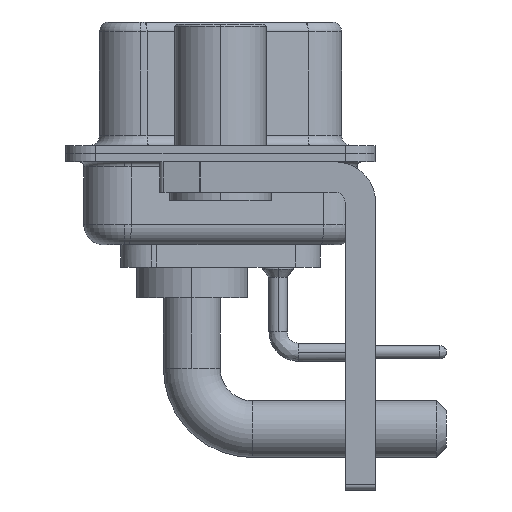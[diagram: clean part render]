
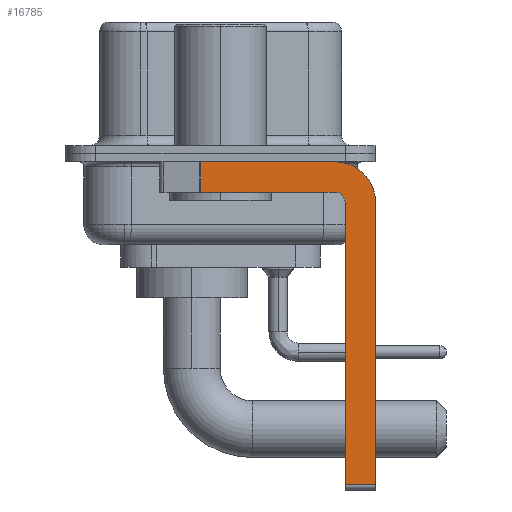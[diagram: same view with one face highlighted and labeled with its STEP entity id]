
A CAD part, left-side view. The second image highlights one B-rep face of the part: STEP entity #16785.
In plain terms, the highlighted planar face has unit normal (-1, 0, 0).
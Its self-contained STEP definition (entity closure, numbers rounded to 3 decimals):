
#169 = CARTESIAN_POINT ( 'NONE',  ( -2.9, -7.65, -16.35 ) ) ;
#586 = DIRECTION ( 'NONE',  ( 0., -1., 0. ) ) ;
#733 = DIRECTION ( 'NONE',  ( 0., 0., -1. ) ) ;
#1070 = VECTOR ( 'NONE', #16345, 1000. ) ;
#1624 = DIRECTION ( 'NONE',  ( 0., 0., -1. ) ) ;
#1710 = LINE ( 'NONE', #3840, #11316 ) ;
#1720 = ORIENTED_EDGE ( 'NONE', *, *, #25575, .F. ) ;
#1809 = VERTEX_POINT ( 'NONE', #169 ) ;
#1882 = LINE ( 'NONE', #2007, #3145 ) ;
#2007 = CARTESIAN_POINT ( 'NONE',  ( -2.9, 0.978, -1.9 ) ) ;
#2187 = LINE ( 'NONE', #10074, #1070 ) ;
#2550 = DIRECTION ( 'NONE',  ( 0., 0., -1. ) ) ;
#2875 = CARTESIAN_POINT ( 'NONE',  ( -2.9, 0.978, -1.9 ) ) ;
#2975 = EDGE_CURVE ( 'NONE', #8226, #8462, #8981, .T. ) ;
#3145 = VECTOR ( 'NONE', #1624, 1000. ) ;
#3410 = EDGE_CURVE ( 'NONE', #8462, #1809, #12719, .T. ) ;
#3652 = ORIENTED_EDGE ( 'NONE', *, *, #23376, .F. ) ;
#3840 = CARTESIAN_POINT ( 'NONE',  ( -2.9, -6.15, -16.6 ) ) ;
#4251 = VERTEX_POINT ( 'NONE', #16491 ) ;
#4537 = CARTESIAN_POINT ( 'NONE',  ( -2.9, -5.65, -1.9 ) ) ;
#4667 = CARTESIAN_POINT ( 'NONE',  ( -2.9, -5.65, -2.4 ) ) ;
#4694 = ORIENTED_EDGE ( 'NONE', *, *, #2975, .F. ) ;
#4807 = PLANE ( 'NONE',  #24754 ) ;
#5439 = VERTEX_POINT ( 'NONE', #19855 ) ;
#5777 = ORIENTED_EDGE ( 'NONE', *, *, #9506, .T. ) ;
#5947 = EDGE_CURVE ( 'NONE', #5439, #8226, #18345, .T. ) ;
#6827 = VERTEX_POINT ( 'NONE', #14478 ) ;
#7837 = DIRECTION ( 'NONE',  ( 0., 0., 1. ) ) ;
#8226 = VERTEX_POINT ( 'NONE', #11596 ) ;
#8462 = VERTEX_POINT ( 'NONE', #9167 ) ;
#8472 = CARTESIAN_POINT ( 'NONE',  ( -2.9, -5.65, -1.9 ) ) ;
#8522 = EDGE_LOOP ( 'NONE', ( #10389, #18802, #3652, #11098, #1720, #5777, #12373, #4694 ) ) ;
#8981 = CIRCLE ( 'NONE', #19205, 2. ) ;
#9109 = VERTEX_POINT ( 'NONE', #2875 ) ;
#9167 = CARTESIAN_POINT ( 'NONE',  ( -2.9, -7.65, -2.4 ) ) ;
#9506 = EDGE_CURVE ( 'NONE', #4251, #1809, #2187, .T. ) ;
#10074 = CARTESIAN_POINT ( 'NONE',  ( -2.9, -5.65, -16.35 ) ) ;
#10216 = DIRECTION ( 'NONE',  ( 0., 1., 0. ) ) ;
#10389 = ORIENTED_EDGE ( 'NONE', *, *, #5947, .F. ) ;
#11098 = ORIENTED_EDGE ( 'NONE', *, *, #25299, .F. ) ;
#11316 = VECTOR ( 'NONE', #7837, 1000. ) ;
#11596 = CARTESIAN_POINT ( 'NONE',  ( -2.9, -5.65, -0.4 ) ) ;
#12373 = ORIENTED_EDGE ( 'NONE', *, *, #3410, .F. ) ;
#12719 = LINE ( 'NONE', #20850, #14964 ) ;
#12869 = CARTESIAN_POINT ( 'NONE',  ( -2.9, 3., -0.4 ) ) ;
#14478 = CARTESIAN_POINT ( 'NONE',  ( -2.9, -6.15, -2.4 ) ) ;
#14545 = DIRECTION ( 'NONE',  ( 0., 0., 1. ) ) ;
#14761 = LINE ( 'NONE', #8472, #24150 ) ;
#14841 = DIRECTION ( 'NONE',  ( 0., 0., -1. ) ) ;
#14964 = VECTOR ( 'NONE', #2550, 1000. ) ;
#15410 = CARTESIAN_POINT ( 'NONE',  ( -2.9, -5.65, -2.4 ) ) ;
#15996 = AXIS2_PLACEMENT_3D ( 'NONE', #16414, #20415, #14545 ) ;
#16345 = DIRECTION ( 'NONE',  ( 0., -1., 0. ) ) ;
#16414 = CARTESIAN_POINT ( 'NONE',  ( -2.9, -5.65, -2.4 ) ) ;
#16491 = CARTESIAN_POINT ( 'NONE',  ( -2.9, -6.15, -16.35 ) ) ;
#16785 = ADVANCED_FACE ( 'NONE', ( #19111 ), #4807, .F. ) ;
#18345 = LINE ( 'NONE', #12869, #20075 ) ;
#18802 = ORIENTED_EDGE ( 'NONE', *, *, #22097, .T. ) ;
#19020 = DIRECTION ( 'NONE',  ( 1., 0., 0. ) ) ;
#19111 = FACE_OUTER_BOUND ( 'NONE', #8522, .T. ) ;
#19205 = AXIS2_PLACEMENT_3D ( 'NONE', #15410, #19020, #733 ) ;
#19380 = DIRECTION ( 'NONE',  ( 1., 0., 0. ) ) ;
#19855 = CARTESIAN_POINT ( 'NONE',  ( -2.9, 0.978, -0.4 ) ) ;
#20075 = VECTOR ( 'NONE', #586, 1000. ) ;
#20415 = DIRECTION ( 'NONE',  ( -1., 0., 0. ) ) ;
#20850 = CARTESIAN_POINT ( 'NONE',  ( -2.9, -7.65, -2.4 ) ) ;
#22097 = EDGE_CURVE ( 'NONE', #5439, #9109, #1882, .T. ) ;
#23376 = EDGE_CURVE ( 'NONE', #23936, #9109, #14761, .T. ) ;
#23936 = VERTEX_POINT ( 'NONE', #4537 ) ;
#24150 = VECTOR ( 'NONE', #10216, 1000. ) ;
#24754 = AXIS2_PLACEMENT_3D ( 'NONE', #4667, #19380, #14841 ) ;
#25299 = EDGE_CURVE ( 'NONE', #6827, #23936, #26234, .T. ) ;
#25575 = EDGE_CURVE ( 'NONE', #4251, #6827, #1710, .T. ) ;
#26234 = CIRCLE ( 'NONE', #15996, 0.5 ) ;
